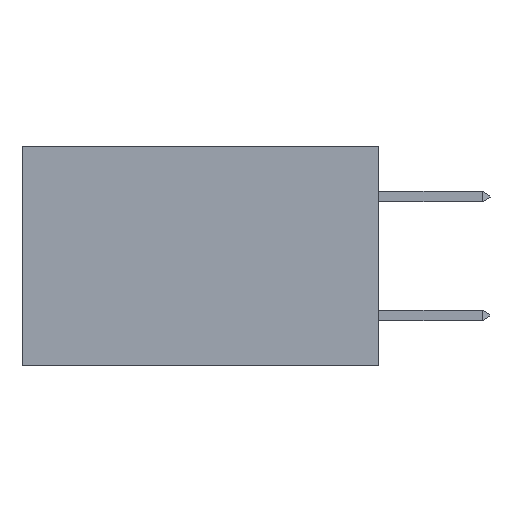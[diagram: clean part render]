
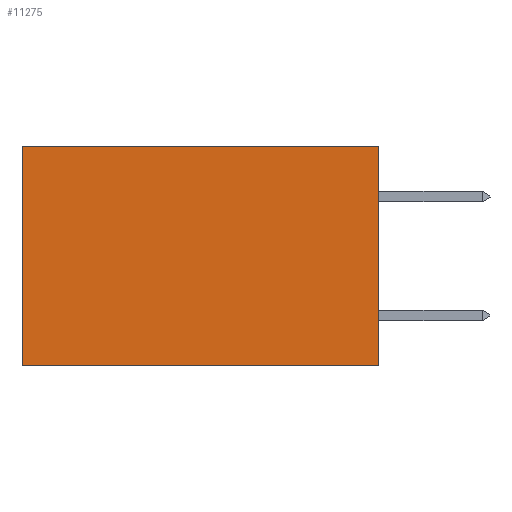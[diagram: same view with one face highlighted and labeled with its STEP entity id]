
A CAD part, left-side view. The second image highlights one B-rep face of the part: STEP entity #11275.
In plain terms, the highlighted planar face has unit normal (-1, 0, 0).
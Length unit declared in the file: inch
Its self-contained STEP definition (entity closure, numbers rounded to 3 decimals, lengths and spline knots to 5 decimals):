
#435 = LINE ( 'NONE', #3262, #3864 ) ;
#450 = VERTEX_POINT ( 'NONE', #15799 ) ;
#1816 = ORIENTED_EDGE ( 'NONE', *, *, #7894, .F. ) ;
#1852 = CARTESIAN_POINT ( 'NONE',  ( 0.298, 0., -0.37 ) ) ;
#2017 = LINE ( 'NONE', #1852, #22125 ) ;
#2323 = CARTESIAN_POINT ( 'NONE',  ( 0.298, 0., 0. ) ) ;
#3262 = CARTESIAN_POINT ( 'NONE',  ( 0.298, 0.6, 0. ) ) ;
#3864 = VECTOR ( 'NONE', #25103, 39.37008 ) ;
#4172 = DIRECTION ( 'NONE',  ( 0., 0., -1. ) ) ;
#4647 = VERTEX_POINT ( 'NONE', #19097 ) ;
#6042 = CARTESIAN_POINT ( 'NONE',  ( 0.298, 0., 0. ) ) ;
#6680 = VERTEX_POINT ( 'NONE', #18667 ) ;
#7665 = LINE ( 'NONE', #23991, #15588 ) ;
#7894 = EDGE_CURVE ( 'NONE', #450, #21953, #2017, .T. ) ;
#8119 = ORIENTED_EDGE ( 'NONE', *, *, #10777, .F. ) ;
#8385 = DIRECTION ( 'NONE',  ( 0., 0., -1. ) ) ;
#8972 = FACE_OUTER_BOUND ( 'NONE', #11353, .T. ) ;
#10777 = EDGE_CURVE ( 'NONE', #6680, #450, #11519, .T. ) ;
#11275 = ADVANCED_FACE ( 'NONE', ( #8972 ), #12516, .F. ) ;
#11353 = EDGE_LOOP ( 'NONE', ( #16494, #1816, #8119, #15218 ) ) ;
#11519 = LINE ( 'NONE', #6042, #25339 ) ;
#11953 = DIRECTION ( 'NONE',  ( 0., 1., 0. ) ) ;
#12255 = DIRECTION ( 'NONE',  ( 1., 0., 0. ) ) ;
#12516 = PLANE ( 'NONE',  #19425 ) ;
#12912 = EDGE_CURVE ( 'NONE', #4647, #21953, #435, .T. ) ;
#14270 = DIRECTION ( 'NONE',  ( 0., 1., 0. ) ) ;
#15218 = ORIENTED_EDGE ( 'NONE', *, *, #17670, .T. ) ;
#15588 = VECTOR ( 'NONE', #14270, 39.37008 ) ;
#15799 = CARTESIAN_POINT ( 'NONE',  ( 0.298, 0., -0.37 ) ) ;
#16494 = ORIENTED_EDGE ( 'NONE', *, *, #12912, .T. ) ;
#17670 = EDGE_CURVE ( 'NONE', #6680, #4647, #7665, .T. ) ;
#18667 = CARTESIAN_POINT ( 'NONE',  ( 0.298, 0., 0. ) ) ;
#19097 = CARTESIAN_POINT ( 'NONE',  ( 0.298, 0.6, 0. ) ) ;
#19425 = AXIS2_PLACEMENT_3D ( 'NONE', #2323, #12255, #4172 ) ;
#19891 = CARTESIAN_POINT ( 'NONE',  ( 0.298, 0.6, -0.37 ) ) ;
#21953 = VERTEX_POINT ( 'NONE', #19891 ) ;
#22125 = VECTOR ( 'NONE', #11953, 39.37008 ) ;
#23991 = CARTESIAN_POINT ( 'NONE',  ( 0.298, 0., 0. ) ) ;
#25103 = DIRECTION ( 'NONE',  ( 0., 0., -1. ) ) ;
#25339 = VECTOR ( 'NONE', #8385, 39.37008 ) ;
